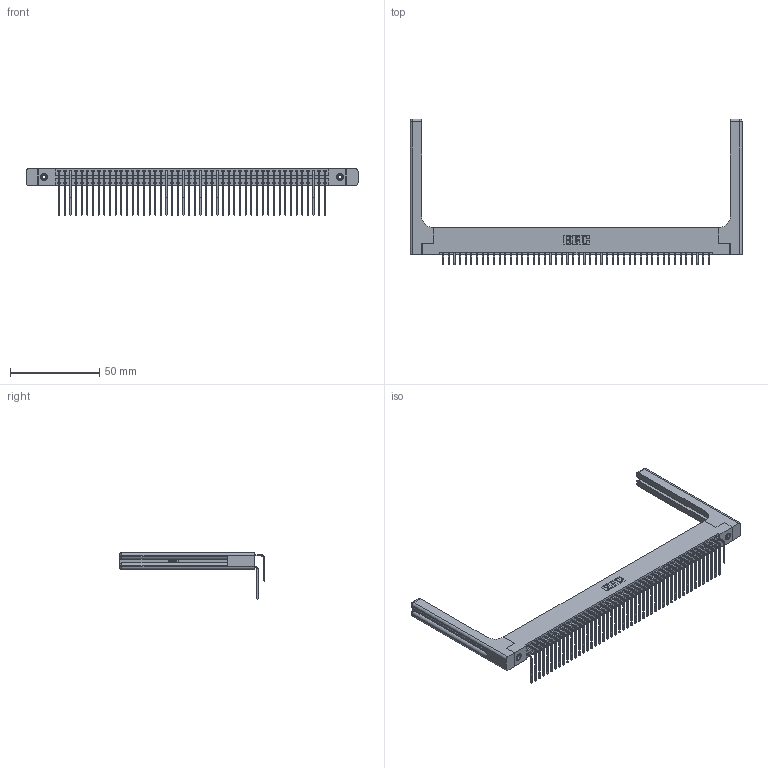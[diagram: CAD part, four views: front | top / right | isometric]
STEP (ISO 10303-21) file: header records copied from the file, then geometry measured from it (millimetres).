
FILE_DESCRIPTION (( 'STEP AP203' ), '1' );
FILE_NAME ('346-096-559-258.STEP', '2022-05-26T17:12:56', ( '' ), ( '' ), 'SwSTEP 2.0', 'SolidWorks 2020', '' );
FILE_SCHEMA (( 'CONFIG_CONTROL_DESIGN' ));
Length unit declared in the file: inch
Products named in the file (6): 345-250-001_345-250-001-102; 345-292-001_559 Tail - 2; 346-096-559-258; 345-292-001_558 559 Tail - 1; 346-220-058_345-220-058; 346 Part_Flush Mounting Lugs - 0.156 Dia-TH
Assembly tree (101 placements, depth 2):
  346-096-559-258
    346 Part_Flush Mounting Lugs - 0.156 Dia-TH
    345-292-001_558 559 Tail - 1  x48
    345-292-001_559 Tail - 2  x48
    345-250-001_345-250-001-102  x2
    346-220-058_345-220-058  x2
Bounding box: 186.46 x 81.85 x 26.16 mm (x, y, z)
Volume: 26258.8 mm3; surface area: 33551.6 mm2
Topology: 101 solids, 101 shells, 5576 faces, 16487 edges, 10842 vertices
Faces by surface type: plane 3790, cylinder 1726, bspline 36, cone 12, sphere 8, torus 4
Entity records: 37900 total; most frequent: CARTESIAN_POINT 7302, ORIENTED_EDGE 5980, DIRECTION 5390, EDGE_CURVE 2990, LINE 2534, VECTOR 2534, VERTEX_POINT 1982, AXIS2_PLACEMENT_3D 1428
